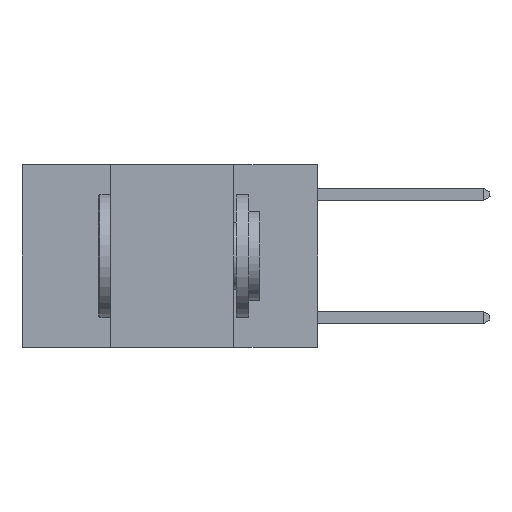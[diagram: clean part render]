
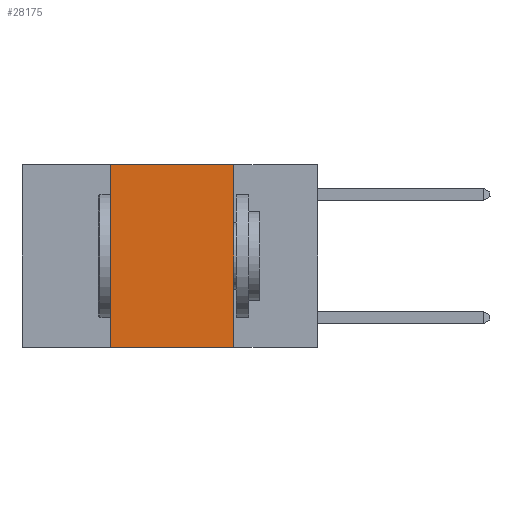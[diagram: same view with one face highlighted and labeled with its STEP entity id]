
A CAD part, left-side view. The second image highlights one B-rep face of the part: STEP entity #28175.
In plain terms, the highlighted planar face has unit normal (-1, 0, 0).
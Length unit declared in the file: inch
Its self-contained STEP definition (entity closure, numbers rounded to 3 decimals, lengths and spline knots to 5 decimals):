
#8 = FACE_OUTER_BOUND ( 'NONE', #1595, .T. ) ;
#476 = DIRECTION ( 'NONE',  ( 1., 0., 0. ) ) ;
#916 = DIRECTION ( 'NONE',  ( 0., -1., 0. ) ) ;
#1002 = EDGE_CURVE ( 'NONE', #13815, #6405, #7294, .T. ) ;
#1387 = LINE ( 'NONE', #27352, #31010 ) ;
#1595 = EDGE_LOOP ( 'NONE', ( #13555, #28945, #11641, #10631 ) ) ;
#3008 = PLANE ( 'NONE',  #26138 ) ;
#3535 = CARTESIAN_POINT ( 'NONE',  ( 0., 0.6, 0. ) ) ;
#5084 = CARTESIAN_POINT ( 'NONE',  ( 0., 0.17, 0. ) ) ;
#6405 = VERTEX_POINT ( 'NONE', #7057 ) ;
#7057 = CARTESIAN_POINT ( 'NONE',  ( 0., 0.17, -0.37 ) ) ;
#7294 = LINE ( 'NONE', #5084, #15215 ) ;
#8439 = EDGE_CURVE ( 'NONE', #29892, #13815, #11123, .T. ) ;
#10181 = VECTOR ( 'NONE', #13503, 39.37008 ) ;
#10187 = CARTESIAN_POINT ( 'NONE',  ( 0., 0.42, 0. ) ) ;
#10396 = EDGE_CURVE ( 'NONE', #16415, #6405, #1387, .T. ) ;
#10631 = ORIENTED_EDGE ( 'NONE', *, *, #10396, .T. ) ;
#11123 = LINE ( 'NONE', #3535, #10181 ) ;
#11531 = CARTESIAN_POINT ( 'NONE',  ( 0., 0.42, 0. ) ) ;
#11641 = ORIENTED_EDGE ( 'NONE', *, *, #12495, .F. ) ;
#12258 = LINE ( 'NONE', #10187, #13909 ) ;
#12495 = EDGE_CURVE ( 'NONE', #16415, #29892, #12258, .T. ) ;
#12513 = DIRECTION ( 'NONE',  ( 0., 0., -1. ) ) ;
#13503 = DIRECTION ( 'NONE',  ( 0., -1., 0. ) ) ;
#13555 = ORIENTED_EDGE ( 'NONE', *, *, #1002, .F. ) ;
#13815 = VERTEX_POINT ( 'NONE', #18098 ) ;
#13909 = VECTOR ( 'NONE', #28876, 39.37008 ) ;
#14594 = DIRECTION ( 'NONE',  ( 0., 0., -1. ) ) ;
#14722 = CARTESIAN_POINT ( 'NONE',  ( 0., 0.6, 0. ) ) ;
#15215 = VECTOR ( 'NONE', #14594, 39.37008 ) ;
#16415 = VERTEX_POINT ( 'NONE', #22267 ) ;
#18098 = CARTESIAN_POINT ( 'NONE',  ( 0., 0.17, 0. ) ) ;
#22267 = CARTESIAN_POINT ( 'NONE',  ( 0., 0.42, -0.37 ) ) ;
#26138 = AXIS2_PLACEMENT_3D ( 'NONE', #14722, #476, #12513 ) ;
#27352 = CARTESIAN_POINT ( 'NONE',  ( 0., 0.6, -0.37 ) ) ;
#28175 = ADVANCED_FACE ( 'NONE', ( #8 ), #3008, .F. ) ;
#28876 = DIRECTION ( 'NONE',  ( 0., 0., 1. ) ) ;
#28945 = ORIENTED_EDGE ( 'NONE', *, *, #8439, .F. ) ;
#29892 = VERTEX_POINT ( 'NONE', #11531 ) ;
#31010 = VECTOR ( 'NONE', #916, 39.37008 ) ;
